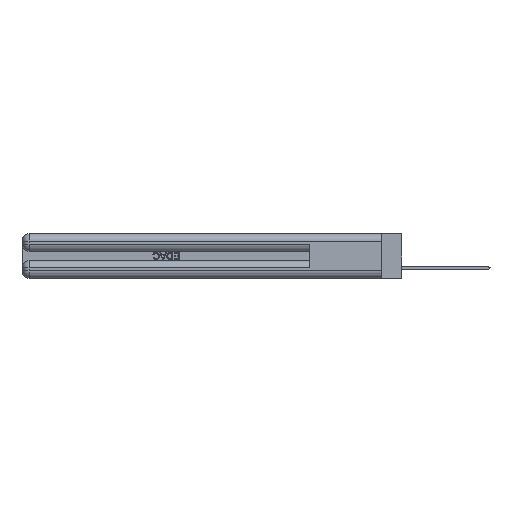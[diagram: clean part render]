
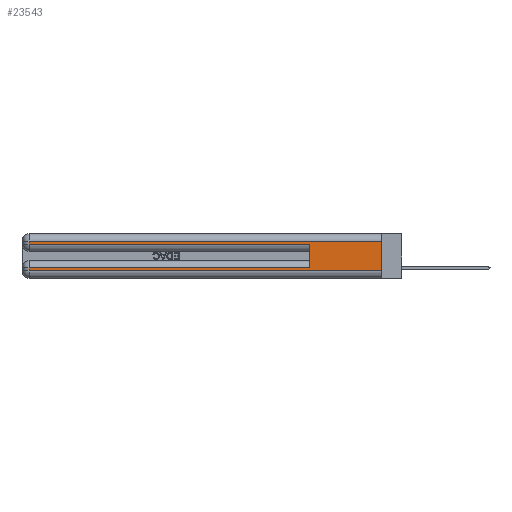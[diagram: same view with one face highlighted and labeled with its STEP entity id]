
A CAD part, left-side view. The second image highlights one B-rep face of the part: STEP entity #23543.
In plain terms, the highlighted planar face has unit normal (-1, 0, 0).
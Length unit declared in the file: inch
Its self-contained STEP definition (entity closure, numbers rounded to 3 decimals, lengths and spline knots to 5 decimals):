
#987 = CARTESIAN_POINT ( 'NONE',  ( 0., 0., 0.37 ) ) ;
#1941 = EDGE_CURVE ( 'NONE', #18422, #13002, #22286, .T. ) ;
#2342 = LINE ( 'NONE', #16751, #15618 ) ;
#2976 = CARTESIAN_POINT ( 'NONE',  ( 0., 0., 0.06 ) ) ;
#3119 = ORIENTED_EDGE ( 'NONE', *, *, #37715, .F. ) ;
#3743 = DIRECTION ( 'NONE',  ( 0., 0., -1. ) ) ;
#4020 = EDGE_CURVE ( 'NONE', #7979, #10344, #18630, .T. ) ;
#5306 = ORIENTED_EDGE ( 'NONE', *, *, #1941, .T. ) ;
#7416 = CARTESIAN_POINT ( 'NONE',  ( 0., 0.6, 0.285 ) ) ;
#7911 = CARTESIAN_POINT ( 'NONE',  ( 0., 0., 0.085 ) ) ;
#7979 = VERTEX_POINT ( 'NONE', #34053 ) ;
#8839 = CARTESIAN_POINT ( 'NONE',  ( 0., 0., 0.06 ) ) ;
#9053 = VECTOR ( 'NONE', #28865, 39.37008 ) ;
#9454 = LINE ( 'NONE', #10028, #21657 ) ;
#9876 = EDGE_CURVE ( 'NONE', #10261, #18422, #35289, .T. ) ;
#10028 = CARTESIAN_POINT ( 'NONE',  ( 0., 0.6, 0.145 ) ) ;
#10072 = AXIS2_PLACEMENT_3D ( 'NONE', #987, #23770, #17518 ) ;
#10261 = VERTEX_POINT ( 'NONE', #19031 ) ;
#10344 = VERTEX_POINT ( 'NONE', #8839 ) ;
#13002 = VERTEX_POINT ( 'NONE', #7416 ) ;
#13190 = ORIENTED_EDGE ( 'NONE', *, *, #32294, .T. ) ;
#14001 = CARTESIAN_POINT ( 'NONE',  ( 0., 2.94, 0.37 ) ) ;
#14387 = PLANE ( 'NONE',  #10072 ) ;
#14907 = EDGE_LOOP ( 'NONE', ( #21081, #27580, #37635, #5306, #3119, #13190, #39223, #25652 ) ) ;
#15618 = VECTOR ( 'NONE', #3743, 39.37008 ) ;
#16511 = CARTESIAN_POINT ( 'NONE',  ( 0., 0.6, 0.085 ) ) ;
#16751 = CARTESIAN_POINT ( 'NONE',  ( 0., 2.94, 0.37 ) ) ;
#16767 = VECTOR ( 'NONE', #17774, 39.37008 ) ;
#17518 = DIRECTION ( 'NONE',  ( 0., 0., -1. ) ) ;
#17774 = DIRECTION ( 'NONE',  ( 0., 1., 0. ) ) ;
#18422 = VERTEX_POINT ( 'NONE', #38189 ) ;
#18630 = LINE ( 'NONE', #2976, #26204 ) ;
#19031 = CARTESIAN_POINT ( 'NONE',  ( 0., 2.94, 0.31 ) ) ;
#19069 = DIRECTION ( 'NONE',  ( 0., 0., -1. ) ) ;
#20670 = EDGE_CURVE ( 'NONE', #31778, #10344, #20849, .T. ) ;
#20849 = LINE ( 'NONE', #38419, #28479 ) ;
#21081 = ORIENTED_EDGE ( 'NONE', *, *, #20670, .F. ) ;
#21088 = CARTESIAN_POINT ( 'NONE',  ( 0., 0., 0.31 ) ) ;
#21657 = VECTOR ( 'NONE', #26664, 39.37008 ) ;
#22286 = LINE ( 'NONE', #25740, #9053 ) ;
#22514 = VECTOR ( 'NONE', #27343, 39.37008 ) ;
#23543 = ADVANCED_FACE ( 'NONE', ( #25059 ), #14387, .F. ) ;
#23770 = DIRECTION ( 'NONE',  ( 1., 0., 0. ) ) ;
#24260 = CARTESIAN_POINT ( 'NONE',  ( 0., 2.94, 0.085 ) ) ;
#25059 = FACE_OUTER_BOUND ( 'NONE', #14907, .T. ) ;
#25233 = DIRECTION ( 'NONE',  ( 0., 0., -1. ) ) ;
#25652 = ORIENTED_EDGE ( 'NONE', *, *, #4020, .T. ) ;
#25740 = CARTESIAN_POINT ( 'NONE',  ( 0., 0., 0.285 ) ) ;
#25755 = DIRECTION ( 'NONE',  ( 0., -1., 0. ) ) ;
#26204 = VECTOR ( 'NONE', #25755, 39.37008 ) ;
#26331 = EDGE_CURVE ( 'NONE', #32792, #7979, #2342, .T. ) ;
#26664 = DIRECTION ( 'NONE',  ( 0., 0., 1. ) ) ;
#27343 = DIRECTION ( 'NONE',  ( 0., 1., 0. ) ) ;
#27580 = ORIENTED_EDGE ( 'NONE', *, *, #39791, .T. ) ;
#28479 = VECTOR ( 'NONE', #25233, 39.37008 ) ;
#28865 = DIRECTION ( 'NONE',  ( 0., -1., 0. ) ) ;
#31778 = VERTEX_POINT ( 'NONE', #21088 ) ;
#32141 = VERTEX_POINT ( 'NONE', #16511 ) ;
#32294 = EDGE_CURVE ( 'NONE', #32141, #32792, #37210, .T. ) ;
#32792 = VERTEX_POINT ( 'NONE', #24260 ) ;
#34053 = CARTESIAN_POINT ( 'NONE',  ( 0., 2.94, 0.06 ) ) ;
#34741 = VECTOR ( 'NONE', #19069, 39.37008 ) ;
#35289 = LINE ( 'NONE', #14001, #34741 ) ;
#37210 = LINE ( 'NONE', #7911, #16767 ) ;
#37395 = CARTESIAN_POINT ( 'NONE',  ( 0., 0., 0.31 ) ) ;
#37635 = ORIENTED_EDGE ( 'NONE', *, *, #9876, .T. ) ;
#37715 = EDGE_CURVE ( 'NONE', #32141, #13002, #9454, .T. ) ;
#38189 = CARTESIAN_POINT ( 'NONE',  ( 0., 2.94, 0.285 ) ) ;
#38419 = CARTESIAN_POINT ( 'NONE',  ( 0., 0., 0.37 ) ) ;
#38422 = LINE ( 'NONE', #37395, #22514 ) ;
#39223 = ORIENTED_EDGE ( 'NONE', *, *, #26331, .T. ) ;
#39791 = EDGE_CURVE ( 'NONE', #31778, #10261, #38422, .T. ) ;
